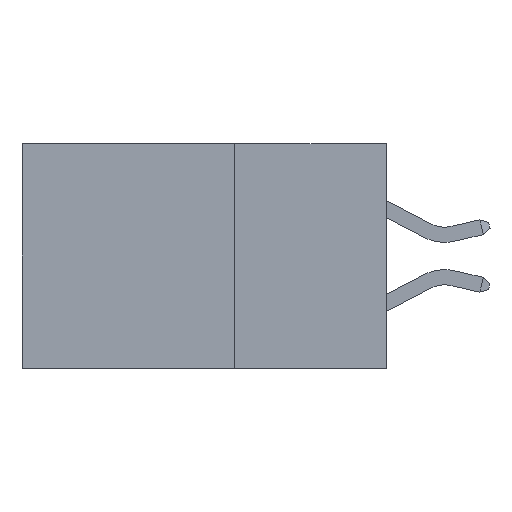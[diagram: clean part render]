
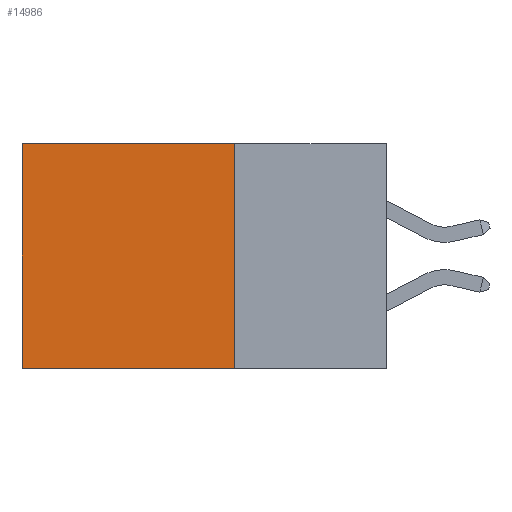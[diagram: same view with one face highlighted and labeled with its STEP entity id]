
A CAD part, left-side view. The second image highlights one B-rep face of the part: STEP entity #14986.
In plain terms, the highlighted planar face has unit normal (-1, 0, 0).
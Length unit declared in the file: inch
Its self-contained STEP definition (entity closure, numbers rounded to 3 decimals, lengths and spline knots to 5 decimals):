
#326 = DIRECTION ( 'NONE',  ( 1., 0., 0. ) ) ;
#749 = DIRECTION ( 'NONE',  ( 0., 1., 0. ) ) ;
#891 = EDGE_CURVE ( 'NONE', #1110, #4964, #9963, .T. ) ;
#1110 = VERTEX_POINT ( 'NONE', #10114 ) ;
#1390 = VERTEX_POINT ( 'NONE', #10798 ) ;
#1877 = DIRECTION ( 'NONE',  ( 0., 1., 0. ) ) ;
#1991 = CARTESIAN_POINT ( 'NONE',  ( 0.298, 0.25, 0. ) ) ;
#2010 = EDGE_LOOP ( 'NONE', ( #5883, #9663, #3331, #11229 ) ) ;
#2074 = CARTESIAN_POINT ( 'NONE',  ( 0.298, 0.6, 0. ) ) ;
#2591 = LINE ( 'NONE', #6152, #8936 ) ;
#2948 = CARTESIAN_POINT ( 'NONE',  ( 0.298, 0.25, 0. ) ) ;
#3266 = EDGE_CURVE ( 'NONE', #7096, #1110, #2591, .T. ) ;
#3331 = ORIENTED_EDGE ( 'NONE', *, *, #8893, .F. ) ;
#4062 = VECTOR ( 'NONE', #1877, 39.37008 ) ;
#4878 = EDGE_CURVE ( 'NONE', #1390, #4964, #7431, .T. ) ;
#4964 = VERTEX_POINT ( 'NONE', #8742 ) ;
#5318 = PLANE ( 'NONE',  #8969 ) ;
#5739 = VECTOR ( 'NONE', #11780, 39.37008 ) ;
#5883 = ORIENTED_EDGE ( 'NONE', *, *, #891, .T. ) ;
#6152 = CARTESIAN_POINT ( 'NONE',  ( 0.298, 0.25, 0. ) ) ;
#6649 = DIRECTION ( 'NONE',  ( 0., 0., -1. ) ) ;
#6766 = FACE_OUTER_BOUND ( 'NONE', #2010, .T. ) ;
#7096 = VERTEX_POINT ( 'NONE', #1991 ) ;
#7431 = LINE ( 'NONE', #11775, #4062 ) ;
#7900 = CARTESIAN_POINT ( 'NONE',  ( 0.298, 0.25, 0. ) ) ;
#8742 = CARTESIAN_POINT ( 'NONE',  ( 0.298, 0.6, -0.37 ) ) ;
#8893 = EDGE_CURVE ( 'NONE', #7096, #1390, #11666, .T. ) ;
#8936 = VECTOR ( 'NONE', #749, 39.37008 ) ;
#8969 = AXIS2_PLACEMENT_3D ( 'NONE', #7900, #326, #9171 ) ;
#9171 = DIRECTION ( 'NONE',  ( 0., 0., -1. ) ) ;
#9663 = ORIENTED_EDGE ( 'NONE', *, *, #4878, .F. ) ;
#9963 = LINE ( 'NONE', #2074, #13567 ) ;
#10114 = CARTESIAN_POINT ( 'NONE',  ( 0.298, 0.6, 0. ) ) ;
#10798 = CARTESIAN_POINT ( 'NONE',  ( 0.298, 0.25, -0.37 ) ) ;
#11229 = ORIENTED_EDGE ( 'NONE', *, *, #3266, .T. ) ;
#11666 = LINE ( 'NONE', #2948, #5739 ) ;
#11775 = CARTESIAN_POINT ( 'NONE',  ( 0.298, 0.25, -0.37 ) ) ;
#11780 = DIRECTION ( 'NONE',  ( 0., 0., -1. ) ) ;
#13567 = VECTOR ( 'NONE', #6649, 39.37008 ) ;
#14986 = ADVANCED_FACE ( 'NONE', ( #6766 ), #5318, .F. ) ;
